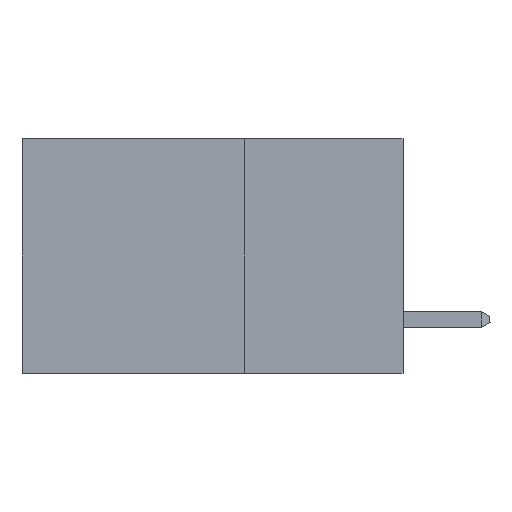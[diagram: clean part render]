
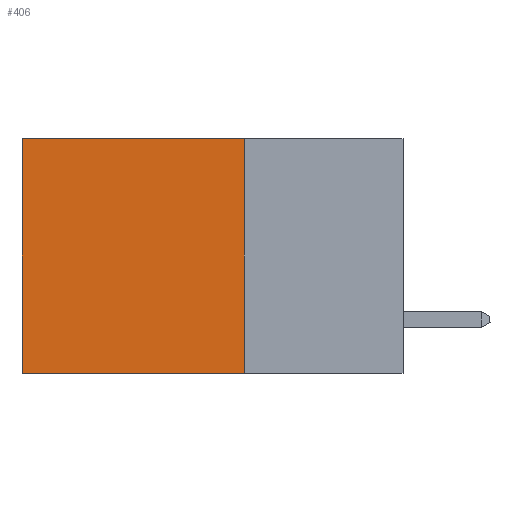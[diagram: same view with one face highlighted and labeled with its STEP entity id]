
A CAD part, left-side view. The second image highlights one B-rep face of the part: STEP entity #406.
In plain terms, the highlighted planar face has unit normal (-1, 0, 0).
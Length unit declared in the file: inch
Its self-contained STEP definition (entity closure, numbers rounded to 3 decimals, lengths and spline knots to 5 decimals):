
#406 = ADVANCED_FACE ( 'NONE', ( #680 ), #1641, .F. ) ;
#574 = CARTESIAN_POINT ( 'NONE',  ( 0.2875, 0.25, -0.37 ) ) ;
#680 = FACE_OUTER_BOUND ( 'NONE', #12663, .T. ) ;
#752 = CARTESIAN_POINT ( 'NONE',  ( 0.2875, 0.25, 0. ) ) ;
#1537 = EDGE_CURVE ( 'NONE', #22697, #1812, #9846, .T. ) ;
#1641 = PLANE ( 'NONE',  #22097 ) ;
#1812 = VERTEX_POINT ( 'NONE', #22486 ) ;
#2444 = ORIENTED_EDGE ( 'NONE', *, *, #12160, .T. ) ;
#2775 = VECTOR ( 'NONE', #10016, 39.37008 ) ;
#5299 = DIRECTION ( 'NONE',  ( 1., 0., 0. ) ) ;
#5407 = VECTOR ( 'NONE', #23413, 39.37008 ) ;
#5482 = CARTESIAN_POINT ( 'NONE',  ( 0.2875, 0.25, 0. ) ) ;
#6267 = ORIENTED_EDGE ( 'NONE', *, *, #1537, .T. ) ;
#6454 = DIRECTION ( 'NONE',  ( 0., 1., 0. ) ) ;
#6711 = EDGE_CURVE ( 'NONE', #26103, #1812, #10436, .T. ) ;
#7110 = ORIENTED_EDGE ( 'NONE', *, *, #11040, .F. ) ;
#7505 = CARTESIAN_POINT ( 'NONE',  ( 0.2875, 0.25, 0. ) ) ;
#9846 = LINE ( 'NONE', #15452, #21182 ) ;
#10016 = DIRECTION ( 'NONE',  ( 0., 1., 0. ) ) ;
#10436 = LINE ( 'NONE', #574, #16896 ) ;
#10566 = LINE ( 'NONE', #752, #5407 ) ;
#11040 = EDGE_CURVE ( 'NONE', #20981, #26103, #10566, .T. ) ;
#11578 = DIRECTION ( 'NONE',  ( 0., 0., -1. ) ) ;
#12160 = EDGE_CURVE ( 'NONE', #20981, #22697, #23721, .T. ) ;
#12431 = CARTESIAN_POINT ( 'NONE',  ( 0.2875, 0.25, 0. ) ) ;
#12663 = EDGE_LOOP ( 'NONE', ( #6267, #14424, #7110, #2444 ) ) ;
#12762 = CARTESIAN_POINT ( 'NONE',  ( 0.2875, 0.6, 0. ) ) ;
#14424 = ORIENTED_EDGE ( 'NONE', *, *, #6711, .F. ) ;
#15452 = CARTESIAN_POINT ( 'NONE',  ( 0.2875, 0.6, 0. ) ) ;
#16828 = DIRECTION ( 'NONE',  ( 0., 0., -1. ) ) ;
#16896 = VECTOR ( 'NONE', #6454, 39.37008 ) ;
#20981 = VERTEX_POINT ( 'NONE', #7505 ) ;
#21182 = VECTOR ( 'NONE', #16828, 39.37008 ) ;
#22097 = AXIS2_PLACEMENT_3D ( 'NONE', #5482, #5299, #11578 ) ;
#22486 = CARTESIAN_POINT ( 'NONE',  ( 0.2875, 0.6, -0.37 ) ) ;
#22697 = VERTEX_POINT ( 'NONE', #12762 ) ;
#23413 = DIRECTION ( 'NONE',  ( 0., 0., -1. ) ) ;
#23721 = LINE ( 'NONE', #12431, #2775 ) ;
#25220 = CARTESIAN_POINT ( 'NONE',  ( 0.2875, 0.25, -0.37 ) ) ;
#26103 = VERTEX_POINT ( 'NONE', #25220 ) ;
